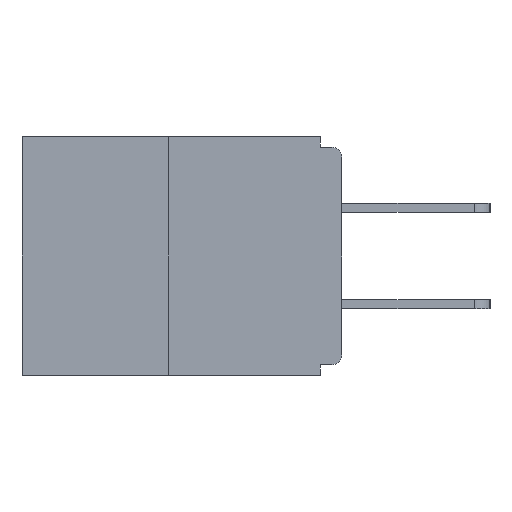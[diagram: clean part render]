
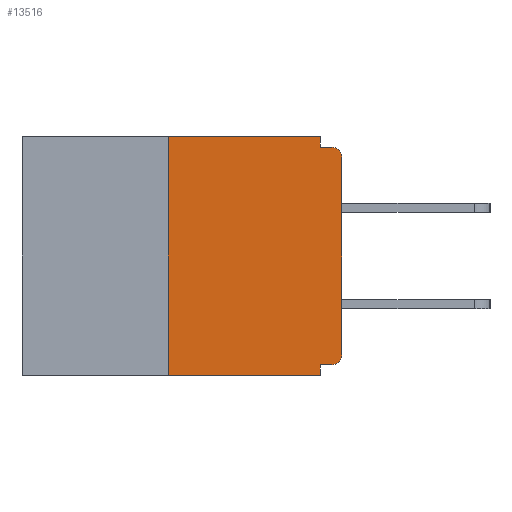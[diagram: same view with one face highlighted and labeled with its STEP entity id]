
A CAD part, left-side view. The second image highlights one B-rep face of the part: STEP entity #13516.
In plain terms, the highlighted planar face has unit normal (-1, 0, 0).
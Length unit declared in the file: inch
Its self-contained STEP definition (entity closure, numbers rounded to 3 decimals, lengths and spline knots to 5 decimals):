
#29 = VERTEX_POINT ( 'NONE', #6733 ) ;
#647 = EDGE_CURVE ( 'NONE', #11961, #14737, #4955, .T. ) ;
#1141 = FACE_OUTER_BOUND ( 'NONE', #9687, .T. ) ;
#1504 = ORIENTED_EDGE ( 'NONE', *, *, #21369, .F. ) ;
#2007 = EDGE_CURVE ( 'NONE', #8215, #24318, #16364, .T. ) ;
#2568 = CARTESIAN_POINT ( 'NONE',  ( 0., 0.031, -0.343 ) ) ;
#3168 = CARTESIAN_POINT ( 'NONE',  ( 0., 0.25, 0. ) ) ;
#3475 = DIRECTION ( 'NONE',  ( 0., -1., 0. ) ) ;
#3862 = DIRECTION ( 'NONE',  ( 0., 0., 1. ) ) ;
#3870 = CARTESIAN_POINT ( 'NONE',  ( 0., 0., -0.313 ) ) ;
#3980 = VERTEX_POINT ( 'NONE', #5245 ) ;
#4177 = EDGE_CURVE ( 'NONE', #22408, #26305, #17494, .T. ) ;
#4546 = EDGE_CURVE ( 'NONE', #8215, #29, #17169, .T. ) ;
#4955 = LINE ( 'NONE', #11483, #25841 ) ;
#5245 = CARTESIAN_POINT ( 'NONE',  ( 0., 0.015, -0.015 ) ) ;
#5265 = DIRECTION ( 'NONE',  ( 0., -1., 0. ) ) ;
#6380 = DIRECTION ( 'NONE',  ( 0., 0., -1. ) ) ;
#6625 = ORIENTED_EDGE ( 'NONE', *, *, #20714, .T. ) ;
#6733 = CARTESIAN_POINT ( 'NONE',  ( 0., 0.031, -0.328 ) ) ;
#7049 = VECTOR ( 'NONE', #7212, 39.37008 ) ;
#7212 = DIRECTION ( 'NONE',  ( 0., 0., 1. ) ) ;
#7636 = EDGE_CURVE ( 'NONE', #26305, #3980, #20284, .T. ) ;
#8197 = LINE ( 'NONE', #15124, #16226 ) ;
#8215 = VERTEX_POINT ( 'NONE', #26666 ) ;
#8998 = AXIS2_PLACEMENT_3D ( 'NONE', #22111, #21961, #19376 ) ;
#9297 = DIRECTION ( 'NONE',  ( 0., -1., 0. ) ) ;
#9320 = ORIENTED_EDGE ( 'NONE', *, *, #4546, .F. ) ;
#9385 = LINE ( 'NONE', #3168, #7049 ) ;
#9687 = EDGE_LOOP ( 'NONE', ( #19326, #1504, #25593, #25027, #9320, #19177, #6625, #11780, #10102, #20110 ) ) ;
#10069 = AXIS2_PLACEMENT_3D ( 'NONE', #25769, #19303, #25918 ) ;
#10102 = ORIENTED_EDGE ( 'NONE', *, *, #7636, .F. ) ;
#10156 = CARTESIAN_POINT ( 'NONE',  ( 0., 0.031, -0.015 ) ) ;
#10533 = VERTEX_POINT ( 'NONE', #23363 ) ;
#11483 = CARTESIAN_POINT ( 'NONE',  ( 0., 0.46, -0.343 ) ) ;
#11629 = AXIS2_PLACEMENT_3D ( 'NONE', #18891, #14412, #18469 ) ;
#11780 = ORIENTED_EDGE ( 'NONE', *, *, #25400, .T. ) ;
#11961 = VERTEX_POINT ( 'NONE', #17955 ) ;
#12247 = VECTOR ( 'NONE', #5265, 39.37008 ) ;
#12701 = CARTESIAN_POINT ( 'NONE',  ( 0., 0., -0.328 ) ) ;
#13516 = ADVANCED_FACE ( 'NONE', ( #1141 ), #20758, .F. ) ;
#14217 = VECTOR ( 'NONE', #24471, 39.37008 ) ;
#14412 = DIRECTION ( 'NONE',  ( 1., 0., 0. ) ) ;
#14737 = VERTEX_POINT ( 'NONE', #24003 ) ;
#14900 = VECTOR ( 'NONE', #6380, 39.37008 ) ;
#15124 = CARTESIAN_POINT ( 'NONE',  ( 0., 0., 0. ) ) ;
#16226 = VECTOR ( 'NONE', #3862, 39.37008 ) ;
#16364 = CIRCLE ( 'NONE', #8998, 0.015 ) ;
#16565 = VERTEX_POINT ( 'NONE', #24407 ) ;
#17169 = LINE ( 'NONE', #12701, #19058 ) ;
#17494 = LINE ( 'NONE', #19368, #14900 ) ;
#17955 = CARTESIAN_POINT ( 'NONE',  ( 0., 0.25, -0.343 ) ) ;
#18469 = DIRECTION ( 'NONE',  ( 0., 0., -1. ) ) ;
#18828 = EDGE_CURVE ( 'NONE', #29, #14737, #20167, .T. ) ;
#18891 = CARTESIAN_POINT ( 'NONE',  ( 0., 0.46, 0. ) ) ;
#19058 = VECTOR ( 'NONE', #23653, 39.37008 ) ;
#19177 = ORIENTED_EDGE ( 'NONE', *, *, #2007, .T. ) ;
#19303 = DIRECTION ( 'NONE',  ( -1., 0., 0. ) ) ;
#19326 = ORIENTED_EDGE ( 'NONE', *, *, #27369, .F. ) ;
#19368 = CARTESIAN_POINT ( 'NONE',  ( 0., 0.031, 0. ) ) ;
#19376 = DIRECTION ( 'NONE',  ( 0., 0., -1. ) ) ;
#20110 = ORIENTED_EDGE ( 'NONE', *, *, #4177, .F. ) ;
#20167 = LINE ( 'NONE', #2568, #14217 ) ;
#20284 = LINE ( 'NONE', #25026, #12247 ) ;
#20714 = EDGE_CURVE ( 'NONE', #24318, #16565, #8197, .T. ) ;
#20758 = PLANE ( 'NONE',  #11629 ) ;
#21369 = EDGE_CURVE ( 'NONE', #11961, #10533, #9385, .T. ) ;
#21961 = DIRECTION ( 'NONE',  ( -1., 0., 0. ) ) ;
#22111 = CARTESIAN_POINT ( 'NONE',  ( 0., 0.015, -0.313 ) ) ;
#22408 = VERTEX_POINT ( 'NONE', #25019 ) ;
#23228 = CARTESIAN_POINT ( 'NONE',  ( 0., 0.46, 0. ) ) ;
#23363 = CARTESIAN_POINT ( 'NONE',  ( 0., 0.25, 0. ) ) ;
#23653 = DIRECTION ( 'NONE',  ( 0., 1., 0. ) ) ;
#24003 = CARTESIAN_POINT ( 'NONE',  ( 0., 0.031, -0.343 ) ) ;
#24318 = VERTEX_POINT ( 'NONE', #3870 ) ;
#24407 = CARTESIAN_POINT ( 'NONE',  ( 0., 0., -0.03 ) ) ;
#24412 = VECTOR ( 'NONE', #3475, 39.37008 ) ;
#24471 = DIRECTION ( 'NONE',  ( 0., 0., -1. ) ) ;
#25019 = CARTESIAN_POINT ( 'NONE',  ( 0., 0.031, 0. ) ) ;
#25026 = CARTESIAN_POINT ( 'NONE',  ( 0., 0., -0.015 ) ) ;
#25027 = ORIENTED_EDGE ( 'NONE', *, *, #18828, .F. ) ;
#25115 = LINE ( 'NONE', #23228, #24412 ) ;
#25400 = EDGE_CURVE ( 'NONE', #16565, #3980, #25695, .T. ) ;
#25593 = ORIENTED_EDGE ( 'NONE', *, *, #647, .T. ) ;
#25695 = CIRCLE ( 'NONE', #10069, 0.015 ) ;
#25769 = CARTESIAN_POINT ( 'NONE',  ( 0., 0.015, -0.03 ) ) ;
#25841 = VECTOR ( 'NONE', #9297, 39.37008 ) ;
#25918 = DIRECTION ( 'NONE',  ( 0., 0., -1. ) ) ;
#26305 = VERTEX_POINT ( 'NONE', #10156 ) ;
#26666 = CARTESIAN_POINT ( 'NONE',  ( 0., 0.015, -0.328 ) ) ;
#27369 = EDGE_CURVE ( 'NONE', #10533, #22408, #25115, .T. ) ;
